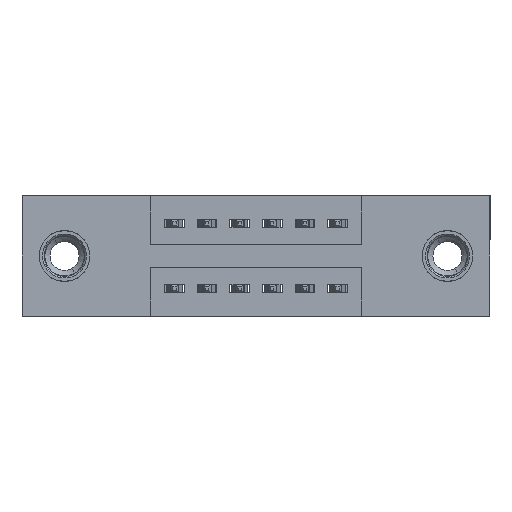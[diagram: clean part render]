
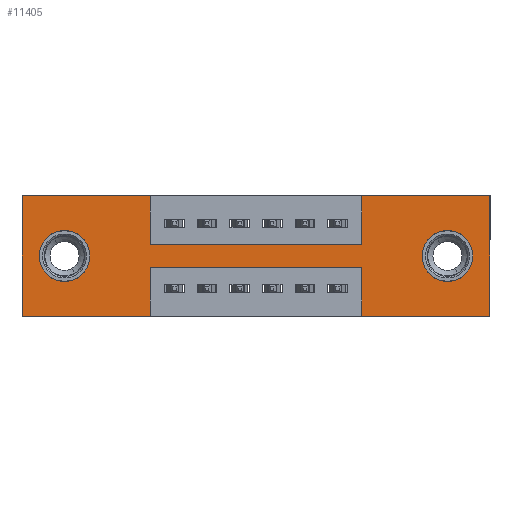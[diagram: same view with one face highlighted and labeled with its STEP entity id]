
A CAD part, front view. The second image highlights one B-rep face of the part: STEP entity #11405.
In plain terms, the highlighted planar face has unit normal (0, -1, 0).
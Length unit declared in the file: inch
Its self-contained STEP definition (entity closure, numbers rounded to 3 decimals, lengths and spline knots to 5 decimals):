
#98 = EDGE_CURVE ( 'NONE', #11972, #365, #7958, .T. ) ;
#233 = VECTOR ( 'NONE', #9853, 39.37008 ) ;
#365 = VERTEX_POINT ( 'NONE', #604 ) ;
#411 = VECTOR ( 'NONE', #6013, 39.37008 ) ;
#604 = CARTESIAN_POINT ( 'NONE',  ( 0., 0., -0.37 ) ) ;
#778 = FACE_BOUND ( 'NONE', #8004, .T. ) ;
#799 = EDGE_CURVE ( 'NONE', #14095, #11760, #5458, .T. ) ;
#832 = VECTOR ( 'NONE', #12489, 39.37008 ) ;
#841 = ORIENTED_EDGE ( 'NONE', *, *, #12522, .F. ) ;
#867 = CARTESIAN_POINT ( 'NONE',  ( 0., 0., 0. ) ) ;
#898 = CARTESIAN_POINT ( 'NONE',  ( 1.305, 0., -0.107 ) ) ;
#1064 = ORIENTED_EDGE ( 'NONE', *, *, #2899, .F. ) ;
#1225 = EDGE_CURVE ( 'NONE', #4349, #3590, #6150, .T. ) ;
#1313 = VECTOR ( 'NONE', #1873, 39.37008 ) ;
#1349 = ORIENTED_EDGE ( 'NONE', *, *, #2921, .F. ) ;
#1668 = CARTESIAN_POINT ( 'NONE',  ( 0.13, 0., -0.263 ) ) ;
#1871 = LINE ( 'NONE', #3709, #13303 ) ;
#1873 = DIRECTION ( 'NONE',  ( 1., 0., 0. ) ) ;
#1955 = CARTESIAN_POINT ( 'NONE',  ( 1.0425, 0., -0.22 ) ) ;
#2160 = CARTESIAN_POINT ( 'NONE',  ( 0.13, 0., -0.185 ) ) ;
#2196 = CARTESIAN_POINT ( 'NONE',  ( 1.435, 0., 0. ) ) ;
#2341 = ORIENTED_EDGE ( 'NONE', *, *, #5708, .F. ) ;
#2669 = AXIS2_PLACEMENT_3D ( 'NONE', #10726, #4074, #11797 ) ;
#2687 = EDGE_CURVE ( 'NONE', #11760, #14095, #9745, .T. ) ;
#2692 = LINE ( 'NONE', #12496, #8357 ) ;
#2899 = EDGE_CURVE ( 'NONE', #6865, #8710, #10247, .T. ) ;
#2921 = EDGE_CURVE ( 'NONE', #8710, #6657, #9909, .T. ) ;
#3031 = DIRECTION ( 'NONE',  ( 0., 0., 1. ) ) ;
#3130 = DIRECTION ( 'NONE',  ( 0., 1., 0. ) ) ;
#3202 = DIRECTION ( 'NONE',  ( 0., 1., 0. ) ) ;
#3513 = AXIS2_PLACEMENT_3D ( 'NONE', #10329, #3646, #11408 ) ;
#3528 = EDGE_CURVE ( 'NONE', #3590, #4349, #9550, .T. ) ;
#3590 = VERTEX_POINT ( 'NONE', #898 ) ;
#3639 = CARTESIAN_POINT ( 'NONE',  ( 1.0425, 0., -0.37 ) ) ;
#3646 = DIRECTION ( 'NONE',  ( 0., 1., 0. ) ) ;
#3709 = CARTESIAN_POINT ( 'NONE',  ( 1.0425, 0., 0. ) ) ;
#3787 = FACE_BOUND ( 'NONE', #6745, .T. ) ;
#3794 = CARTESIAN_POINT ( 'NONE',  ( 0.3925, 0., -0.37 ) ) ;
#3843 = LINE ( 'NONE', #11417, #832 ) ;
#3895 = ORIENTED_EDGE ( 'NONE', *, *, #4790, .F. ) ;
#3939 = CARTESIAN_POINT ( 'NONE',  ( 1.435, 0., -0.37 ) ) ;
#4074 = DIRECTION ( 'NONE',  ( 0., 1., 0. ) ) ;
#4334 = VECTOR ( 'NONE', #12844, 39.37008 ) ;
#4349 = VERTEX_POINT ( 'NONE', #12022 ) ;
#4496 = VECTOR ( 'NONE', #8349, 39.37008 ) ;
#4539 = CARTESIAN_POINT ( 'NONE',  ( 0.13, 0., -0.107 ) ) ;
#4715 = ORIENTED_EDGE ( 'NONE', *, *, #98, .F. ) ;
#4790 = EDGE_CURVE ( 'NONE', #7786, #5613, #6261, .T. ) ;
#4872 = VERTEX_POINT ( 'NONE', #9957 ) ;
#4941 = VECTOR ( 'NONE', #7622, 39.37008 ) ;
#5013 = LINE ( 'NONE', #5969, #411 ) ;
#5036 = AXIS2_PLACEMENT_3D ( 'NONE', #6131, #6177, #13811 ) ;
#5041 = PLANE ( 'NONE',  #5036 ) ;
#5112 = ORIENTED_EDGE ( 'NONE', *, *, #799, .T. ) ;
#5300 = VERTEX_POINT ( 'NONE', #1955 ) ;
#5334 = ORIENTED_EDGE ( 'NONE', *, *, #5670, .F. ) ;
#5458 = CIRCLE ( 'NONE', #11150, 0.078 ) ;
#5613 = VERTEX_POINT ( 'NONE', #8142 ) ;
#5670 = EDGE_CURVE ( 'NONE', #9630, #10813, #2692, .T. ) ;
#5708 = EDGE_CURVE ( 'NONE', #365, #6865, #5013, .T. ) ;
#5969 = CARTESIAN_POINT ( 'NONE',  ( 0., 0., 0. ) ) ;
#6013 = DIRECTION ( 'NONE',  ( 0., 0., 1. ) ) ;
#6061 = CARTESIAN_POINT ( 'NONE',  ( 0.3925, 0., -0.37 ) ) ;
#6131 = CARTESIAN_POINT ( 'NONE',  ( 0., 0., -0.37 ) ) ;
#6150 = CIRCLE ( 'NONE', #13032, 0.078 ) ;
#6177 = DIRECTION ( 'NONE',  ( 0., -1., 0. ) ) ;
#6261 = LINE ( 'NONE', #867, #233 ) ;
#6657 = VERTEX_POINT ( 'NONE', #14226 ) ;
#6745 = EDGE_LOOP ( 'NONE', ( #12302, #11149 ) ) ;
#6865 = VERTEX_POINT ( 'NONE', #13434 ) ;
#6872 = CARTESIAN_POINT ( 'NONE',  ( 0.3925, 0., 0. ) ) ;
#7338 = VECTOR ( 'NONE', #10017, 39.37008 ) ;
#7413 = CARTESIAN_POINT ( 'NONE',  ( 0.3925, 0., -0.15 ) ) ;
#7622 = DIRECTION ( 'NONE',  ( -1., 0., 0. ) ) ;
#7786 = VERTEX_POINT ( 'NONE', #11829 ) ;
#7958 = LINE ( 'NONE', #12972, #4941 ) ;
#7970 = CARTESIAN_POINT ( 'NONE',  ( 1.305, 0., -0.185 ) ) ;
#8004 = EDGE_LOOP ( 'NONE', ( #12476, #5112 ) ) ;
#8142 = CARTESIAN_POINT ( 'NONE',  ( 1.435, 0., 0. ) ) ;
#8164 = DIRECTION ( 'NONE',  ( 0., 0., 1. ) ) ;
#8349 = DIRECTION ( 'NONE',  ( 0., 0., -1. ) ) ;
#8357 = VECTOR ( 'NONE', #13610, 39.37008 ) ;
#8667 = ORIENTED_EDGE ( 'NONE', *, *, #10131, .F. ) ;
#8710 = VERTEX_POINT ( 'NONE', #6872 ) ;
#8828 = EDGE_CURVE ( 'NONE', #5300, #4872, #3843, .T. ) ;
#8865 = ORIENTED_EDGE ( 'NONE', *, *, #8828, .F. ) ;
#9380 = ORIENTED_EDGE ( 'NONE', *, *, #11473, .F. ) ;
#9475 = EDGE_CURVE ( 'NONE', #10813, #5300, #13504, .T. ) ;
#9550 = CIRCLE ( 'NONE', #2669, 0.078 ) ;
#9630 = VERTEX_POINT ( 'NONE', #3939 ) ;
#9745 = CIRCLE ( 'NONE', #3513, 0.078 ) ;
#9853 = DIRECTION ( 'NONE',  ( 1., 0., 0. ) ) ;
#9898 = LINE ( 'NONE', #2196, #7338 ) ;
#9909 = LINE ( 'NONE', #12940, #4334 ) ;
#9956 = VECTOR ( 'NONE', #8164, 39.37008 ) ;
#9957 = CARTESIAN_POINT ( 'NONE',  ( 0.3925, 0., -0.22 ) ) ;
#10017 = DIRECTION ( 'NONE',  ( 0., 0., -1. ) ) ;
#10131 = EDGE_CURVE ( 'NONE', #11556, #7786, #1871, .T. ) ;
#10247 = LINE ( 'NONE', #12892, #1313 ) ;
#10265 = ORIENTED_EDGE ( 'NONE', *, *, #12312, .F. ) ;
#10329 = CARTESIAN_POINT ( 'NONE',  ( 0.13, 0., -0.185 ) ) ;
#10724 = LINE ( 'NONE', #3794, #4496 ) ;
#10726 = CARTESIAN_POINT ( 'NONE',  ( 1.305, 0., -0.185 ) ) ;
#10813 = VERTEX_POINT ( 'NONE', #11144 ) ;
#10921 = DIRECTION ( 'NONE',  ( 0., 0., -1. ) ) ;
#11144 = CARTESIAN_POINT ( 'NONE',  ( 1.0425, 0., -0.37 ) ) ;
#11149 = ORIENTED_EDGE ( 'NONE', *, *, #1225, .T. ) ;
#11150 = AXIS2_PLACEMENT_3D ( 'NONE', #2160, #3202, #3031 ) ;
#11257 = VECTOR ( 'NONE', #12745, 39.37008 ) ;
#11405 = ADVANCED_FACE ( 'NONE', ( #3787, #778, #12261 ), #5041, .T. ) ;
#11408 = DIRECTION ( 'NONE',  ( 0., 0., 1. ) ) ;
#11417 = CARTESIAN_POINT ( 'NONE',  ( 0.3925, 0., -0.22 ) ) ;
#11473 = EDGE_CURVE ( 'NONE', #6657, #11556, #11585, .T. ) ;
#11556 = VERTEX_POINT ( 'NONE', #12928 ) ;
#11585 = LINE ( 'NONE', #7413, #11257 ) ;
#11699 = EDGE_LOOP ( 'NONE', ( #841, #8865, #12998, #5334, #10265, #3895, #8667, #9380, #1349, #1064, #2341, #4715 ) ) ;
#11760 = VERTEX_POINT ( 'NONE', #4539 ) ;
#11797 = DIRECTION ( 'NONE',  ( 0., 0., -1. ) ) ;
#11829 = CARTESIAN_POINT ( 'NONE',  ( 1.0425, 0., 0. ) ) ;
#11972 = VERTEX_POINT ( 'NONE', #6061 ) ;
#12022 = CARTESIAN_POINT ( 'NONE',  ( 1.305, 0., -0.263 ) ) ;
#12261 = FACE_OUTER_BOUND ( 'NONE', #11699, .T. ) ;
#12302 = ORIENTED_EDGE ( 'NONE', *, *, #3528, .T. ) ;
#12312 = EDGE_CURVE ( 'NONE', #5613, #9630, #9898, .T. ) ;
#12476 = ORIENTED_EDGE ( 'NONE', *, *, #2687, .T. ) ;
#12489 = DIRECTION ( 'NONE',  ( -1., 0., 0. ) ) ;
#12496 = CARTESIAN_POINT ( 'NONE',  ( 0., 0., -0.37 ) ) ;
#12522 = EDGE_CURVE ( 'NONE', #4872, #11972, #10724, .T. ) ;
#12745 = DIRECTION ( 'NONE',  ( 1., 0., 0. ) ) ;
#12844 = DIRECTION ( 'NONE',  ( 0., 0., -1. ) ) ;
#12892 = CARTESIAN_POINT ( 'NONE',  ( 0., 0., 0. ) ) ;
#12928 = CARTESIAN_POINT ( 'NONE',  ( 1.0425, 0., -0.15 ) ) ;
#12940 = CARTESIAN_POINT ( 'NONE',  ( 0.3925, 0., 0. ) ) ;
#12972 = CARTESIAN_POINT ( 'NONE',  ( 0., 0., -0.37 ) ) ;
#12998 = ORIENTED_EDGE ( 'NONE', *, *, #9475, .F. ) ;
#13032 = AXIS2_PLACEMENT_3D ( 'NONE', #7970, #3130, #10921 ) ;
#13303 = VECTOR ( 'NONE', #13663, 39.37008 ) ;
#13434 = CARTESIAN_POINT ( 'NONE',  ( 0., 0., 0. ) ) ;
#13504 = LINE ( 'NONE', #3639, #9956 ) ;
#13610 = DIRECTION ( 'NONE',  ( -1., 0., 0. ) ) ;
#13663 = DIRECTION ( 'NONE',  ( 0., 0., 1. ) ) ;
#13811 = DIRECTION ( 'NONE',  ( 0., 0., -1. ) ) ;
#14095 = VERTEX_POINT ( 'NONE', #1668 ) ;
#14226 = CARTESIAN_POINT ( 'NONE',  ( 0.3925, 0., -0.15 ) ) ;
